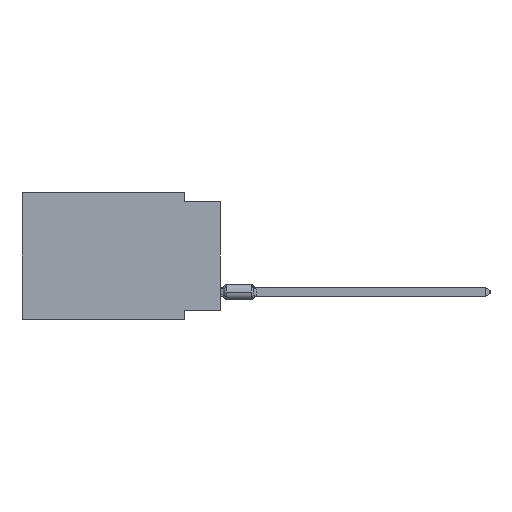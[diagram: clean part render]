
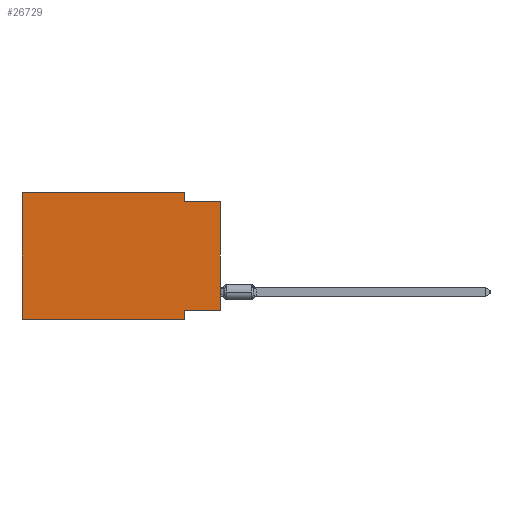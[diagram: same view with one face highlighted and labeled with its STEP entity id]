
A CAD part, left-side view. The second image highlights one B-rep face of the part: STEP entity #26729.
In plain terms, the highlighted planar face has unit normal (-1, 0, 0).
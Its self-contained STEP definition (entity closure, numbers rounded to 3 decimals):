
#1346 = EDGE_CURVE ( 'NONE', #28366, #39947, #19581, .T. ) ;
#3272 = PLANE ( 'NONE',  #18619 ) ;
#4261 = EDGE_CURVE ( 'NONE', #29315, #32030, #33427, .T. ) ;
#4417 = ORIENTED_EDGE ( 'NONE', *, *, #45306, .F. ) ;
#4858 = VERTEX_POINT ( 'NONE', #43531 ) ;
#5433 = VECTOR ( 'NONE', #45173, 1000. ) ;
#5819 = DIRECTION ( 'NONE',  ( 0., -1., 0. ) ) ;
#6066 = LINE ( 'NONE', #9655, #12237 ) ;
#7926 = ORIENTED_EDGE ( 'NONE', *, *, #4261, .T. ) ;
#8072 = CARTESIAN_POINT ( 'NONE',  ( 0., 0., -8.255 ) ) ;
#8316 = DIRECTION ( 'NONE',  ( 0., 1., 0. ) ) ;
#9264 = EDGE_CURVE ( 'NONE', #4858, #21061, #36379, .T. ) ;
#9655 = CARTESIAN_POINT ( 'NONE',  ( 0., 13.97, 0. ) ) ;
#9670 = ORIENTED_EDGE ( 'NONE', *, *, #46369, .F. ) ;
#11967 = ORIENTED_EDGE ( 'NONE', *, *, #26148, .F. ) ;
#12237 = VECTOR ( 'NONE', #5819, 1000. ) ;
#15098 = ORIENTED_EDGE ( 'NONE', *, *, #45657, .F. ) ;
#15293 = DIRECTION ( 'NONE',  ( 1., 0., 0. ) ) ;
#15988 = CARTESIAN_POINT ( 'NONE',  ( 0., 0., -0.635 ) ) ;
#18619 = AXIS2_PLACEMENT_3D ( 'NONE', #50300, #15293, #22712 ) ;
#19581 = LINE ( 'NONE', #8072, #43494 ) ;
#20357 = DIRECTION ( 'NONE',  ( 0., 0., 1. ) ) ;
#21061 = VERTEX_POINT ( 'NONE', #34933 ) ;
#21187 = CARTESIAN_POINT ( 'NONE',  ( 0., 13.97, -8.89 ) ) ;
#21937 = DIRECTION ( 'NONE',  ( 0., 0., 1. ) ) ;
#22712 = DIRECTION ( 'NONE',  ( 0., 0., -1. ) ) ;
#22921 = VECTOR ( 'NONE', #20357, 1000. ) ;
#24753 = CARTESIAN_POINT ( 'NONE',  ( 0., 13.97, -8.89 ) ) ;
#25280 = ORIENTED_EDGE ( 'NONE', *, *, #39978, .T. ) ;
#25608 = CARTESIAN_POINT ( 'NONE',  ( 0., 0., -0.635 ) ) ;
#25631 = DIRECTION ( 'NONE',  ( 0., 0., -1. ) ) ;
#25856 = ORIENTED_EDGE ( 'NONE', *, *, #1346, .F. ) ;
#26131 = CARTESIAN_POINT ( 'NONE',  ( 0., 2.54, -8.89 ) ) ;
#26148 = EDGE_CURVE ( 'NONE', #21061, #41339, #36837, .T. ) ;
#26497 = CARTESIAN_POINT ( 'NONE',  ( 0., 13.97, 0. ) ) ;
#26729 = ADVANCED_FACE ( 'NONE', ( #34690 ), #3272, .F. ) ;
#26771 = LINE ( 'NONE', #41834, #34157 ) ;
#27419 = CARTESIAN_POINT ( 'NONE',  ( 0., 0., -8.255 ) ) ;
#28003 = CARTESIAN_POINT ( 'NONE',  ( 0., 2.54, -8.255 ) ) ;
#28366 = VERTEX_POINT ( 'NONE', #27419 ) ;
#29315 = VERTEX_POINT ( 'NONE', #24753 ) ;
#29490 = DIRECTION ( 'NONE',  ( 0., 0., -1. ) ) ;
#30021 = VECTOR ( 'NONE', #25631, 1000. ) ;
#31575 = DIRECTION ( 'NONE',  ( 0., -1., 0. ) ) ;
#32030 = VERTEX_POINT ( 'NONE', #38256 ) ;
#32702 = EDGE_LOOP ( 'NONE', ( #25280, #11967, #47839, #9670, #15098, #7926, #4417, #25856 ) ) ;
#33427 = LINE ( 'NONE', #21187, #5433 ) ;
#34157 = VECTOR ( 'NONE', #21937, 1000. ) ;
#34690 = FACE_OUTER_BOUND ( 'NONE', #32702, .T. ) ;
#34933 = CARTESIAN_POINT ( 'NONE',  ( 0., 2.54, -0.635 ) ) ;
#36379 = LINE ( 'NONE', #48379, #40711 ) ;
#36837 = LINE ( 'NONE', #15988, #40263 ) ;
#38256 = CARTESIAN_POINT ( 'NONE',  ( 0., 2.54, -8.89 ) ) ;
#39761 = CARTESIAN_POINT ( 'NONE',  ( 0., 0., 0. ) ) ;
#39947 = VERTEX_POINT ( 'NONE', #28003 ) ;
#39978 = EDGE_CURVE ( 'NONE', #28366, #41339, #44096, .T. ) ;
#40263 = VECTOR ( 'NONE', #31575, 1000. ) ;
#40711 = VECTOR ( 'NONE', #29490, 1000. ) ;
#40961 = LINE ( 'NONE', #26131, #30021 ) ;
#41339 = VERTEX_POINT ( 'NONE', #25608 ) ;
#41834 = CARTESIAN_POINT ( 'NONE',  ( 0., 13.97, 0. ) ) ;
#43494 = VECTOR ( 'NONE', #8316, 1000. ) ;
#43531 = CARTESIAN_POINT ( 'NONE',  ( 0., 2.54, 0. ) ) ;
#44096 = LINE ( 'NONE', #39761, #22921 ) ;
#45173 = DIRECTION ( 'NONE',  ( 0., -1., 0. ) ) ;
#45306 = EDGE_CURVE ( 'NONE', #39947, #32030, #40961, .T. ) ;
#45645 = VERTEX_POINT ( 'NONE', #26497 ) ;
#45657 = EDGE_CURVE ( 'NONE', #29315, #45645, #26771, .T. ) ;
#46369 = EDGE_CURVE ( 'NONE', #45645, #4858, #6066, .T. ) ;
#47839 = ORIENTED_EDGE ( 'NONE', *, *, #9264, .F. ) ;
#48379 = CARTESIAN_POINT ( 'NONE',  ( 0., 2.54, 0. ) ) ;
#50300 = CARTESIAN_POINT ( 'NONE',  ( 0., 13.97, 0. ) ) ;
